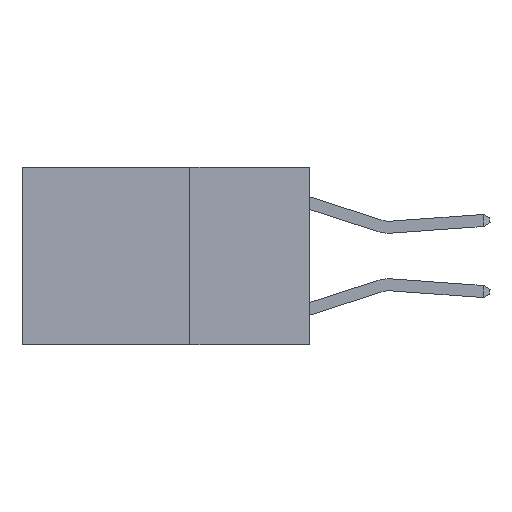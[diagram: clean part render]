
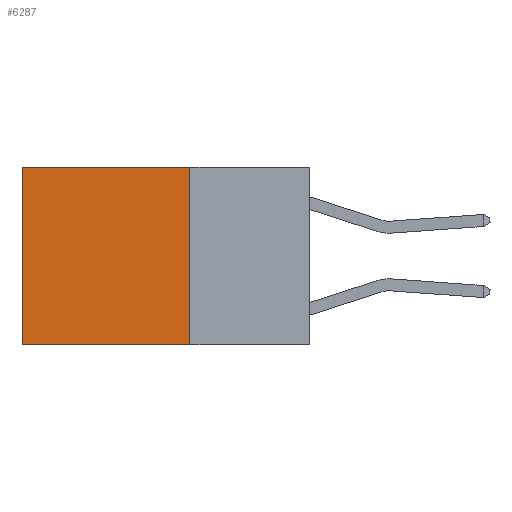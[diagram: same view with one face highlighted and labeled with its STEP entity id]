
A CAD part, left-side view. The second image highlights one B-rep face of the part: STEP entity #6287.
In plain terms, the highlighted planar face has unit normal (-1, 0, 0).
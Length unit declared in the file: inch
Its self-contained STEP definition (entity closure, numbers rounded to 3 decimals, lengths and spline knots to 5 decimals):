
#97 = DIRECTION ( 'NONE',  ( 0., 0., -1. ) ) ;
#882 = DIRECTION ( 'NONE',  ( 0., 1., 0. ) ) ;
#1109 = CARTESIAN_POINT ( 'NONE',  ( 0.2625, 0.6, -0.37 ) ) ;
#1561 = EDGE_CURVE ( 'NONE', #4146, #12653, #13187, .T. ) ;
#2328 = DIRECTION ( 'NONE',  ( 1., 0., 0. ) ) ;
#2430 = LINE ( 'NONE', #6791, #6801 ) ;
#2600 = PLANE ( 'NONE',  #8633 ) ;
#2699 = ORIENTED_EDGE ( 'NONE', *, *, #8785, .F. ) ;
#3036 = VERTEX_POINT ( 'NONE', #1109 ) ;
#3512 = CARTESIAN_POINT ( 'NONE',  ( 0.2625, 0.6, 0. ) ) ;
#3788 = ORIENTED_EDGE ( 'NONE', *, *, #12508, .F. ) ;
#4146 = VERTEX_POINT ( 'NONE', #10382 ) ;
#5372 = VECTOR ( 'NONE', #7939, 39.37008 ) ;
#5709 = DIRECTION ( 'NONE',  ( 0., 1., 0. ) ) ;
#5808 = CARTESIAN_POINT ( 'NONE',  ( 0.2625, 0.6, 0. ) ) ;
#5846 = CARTESIAN_POINT ( 'NONE',  ( 0.2625, 0.25, 0. ) ) ;
#6287 = ADVANCED_FACE ( 'NONE', ( #11452 ), #2600, .F. ) ;
#6791 = CARTESIAN_POINT ( 'NONE',  ( 0.2625, 0.25, 0. ) ) ;
#6801 = VECTOR ( 'NONE', #97, 39.37008 ) ;
#7939 = DIRECTION ( 'NONE',  ( 0., 0., -1. ) ) ;
#8633 = AXIS2_PLACEMENT_3D ( 'NONE', #5846, #2328, #12488 ) ;
#8728 = EDGE_CURVE ( 'NONE', #12653, #3036, #12238, .T. ) ;
#8785 = EDGE_CURVE ( 'NONE', #4146, #14287, #2430, .T. ) ;
#8981 = VECTOR ( 'NONE', #882, 39.37008 ) ;
#9803 = CARTESIAN_POINT ( 'NONE',  ( 0.2625, 0.25, -0.37 ) ) ;
#10382 = CARTESIAN_POINT ( 'NONE',  ( 0.2625, 0.25, 0. ) ) ;
#10449 = ORIENTED_EDGE ( 'NONE', *, *, #1561, .T. ) ;
#10899 = LINE ( 'NONE', #10972, #8981 ) ;
#10972 = CARTESIAN_POINT ( 'NONE',  ( 0.2625, 0.25, -0.37 ) ) ;
#11320 = CARTESIAN_POINT ( 'NONE',  ( 0.2625, 0.25, 0. ) ) ;
#11452 = FACE_OUTER_BOUND ( 'NONE', #12674, .T. ) ;
#12238 = LINE ( 'NONE', #5808, #5372 ) ;
#12488 = DIRECTION ( 'NONE',  ( 0., 0., -1. ) ) ;
#12508 = EDGE_CURVE ( 'NONE', #14287, #3036, #10899, .T. ) ;
#12653 = VERTEX_POINT ( 'NONE', #3512 ) ;
#12674 = EDGE_LOOP ( 'NONE', ( #14363, #3788, #2699, #10449 ) ) ;
#13187 = LINE ( 'NONE', #11320, #13306 ) ;
#13306 = VECTOR ( 'NONE', #5709, 39.37008 ) ;
#14287 = VERTEX_POINT ( 'NONE', #9803 ) ;
#14363 = ORIENTED_EDGE ( 'NONE', *, *, #8728, .T. ) ;
